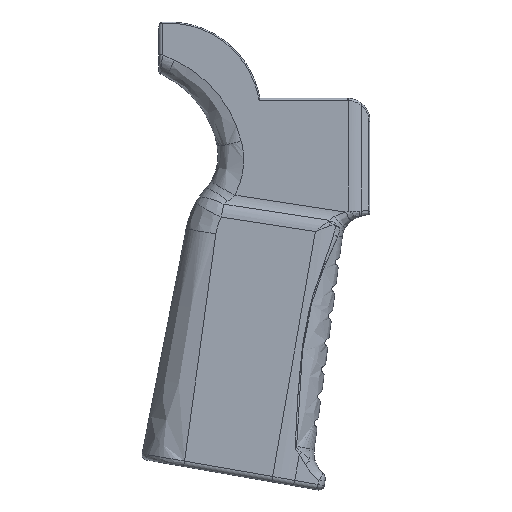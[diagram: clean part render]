
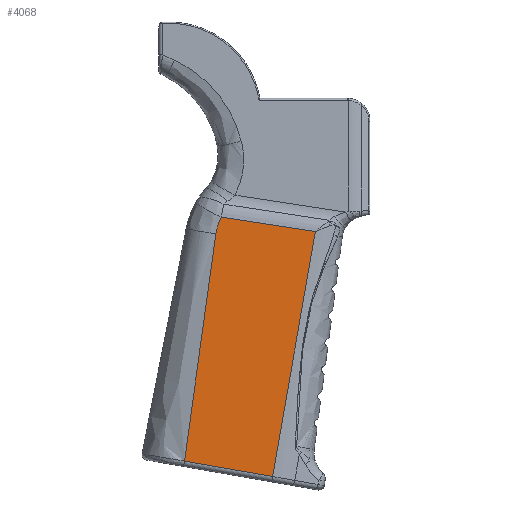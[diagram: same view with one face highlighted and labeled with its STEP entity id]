
A CAD part, left-side view. The second image highlights one B-rep face of the part: STEP entity #4068.
In plain terms, the highlighted planar face has unit normal (-1, 0, 0).
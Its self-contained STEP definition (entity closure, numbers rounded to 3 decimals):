
#224=PLANE('',#4393);
#483=FACE_OUTER_BOUND('',#751,.T.);
#751=EDGE_LOOP('',(#3697,#3698,#3699,#3700,#3701));
#1197=B_SPLINE_CURVE_WITH_KNOTS('',3,(#13325,#13326,#13327,#13328),
 .UNSPECIFIED.,.F.,.F.,(4,4),(6.533,7.017),
 .UNSPECIFIED.);
#1204=B_SPLINE_CURVE_WITH_KNOTS('',3,(#13594,#13595,#13596,#13597),
 .UNSPECIFIED.,.F.,.F.,(4,4),(0.175,6.533),
 .UNSPECIFIED.);
#1363=LINE('',#13222,#1530);
#1365=LINE('',#13591,#1532);
#1366=LINE('',#13593,#1533);
#1530=VECTOR('',#5151,10.);
#1532=VECTOR('',#5163,10.);
#1533=VECTOR('',#5166,10.);
#1831=VERTEX_POINT('',#11525);
#1880=VERTEX_POINT('',#12554);
#1899=VERTEX_POINT('',#13216);
#1903=VERTEX_POINT('',#13317);
#1906=VERTEX_POINT('',#13589);
#2499=EDGE_CURVE('',#1899,#1880,#1363,.T.);
#2506=EDGE_CURVE('',#1903,#1899,#1197,.T.);
#2515=EDGE_CURVE('',#1880,#1906,#1365,.T.);
#2516=EDGE_CURVE('',#1906,#1831,#1366,.T.);
#2517=EDGE_CURVE('',#1831,#1903,#1204,.T.);
#3697=ORIENTED_EDGE('',*,*,#2516,.F.);
#3698=ORIENTED_EDGE('',*,*,#2515,.F.);
#3699=ORIENTED_EDGE('',*,*,#2499,.F.);
#3700=ORIENTED_EDGE('',*,*,#2506,.F.);
#3701=ORIENTED_EDGE('',*,*,#2517,.F.);
#4068=ADVANCED_FACE('',(#483),#224,.F.);
#4393=AXIS2_PLACEMENT_3D('',#13592,#5164,#5165);
#5151=DIRECTION('',(0.,-0.989,-0.151));
#5163=DIRECTION('',(0.,0.172,-0.985));
#5164=DIRECTION('center_axis',(1.,0.,0.));
#5165=DIRECTION('ref_axis',(0.,-0.989,-0.151));
#5166=DIRECTION('',(0.,0.985,0.172));
#11525=CARTESIAN_POINT('',(11.668,-98.506,-71.96));
#12554=CARTESIAN_POINT('',(11.668,-134.704,-8.461));
#13216=CARTESIAN_POINT('',(11.668,-108.616,-4.478));
#13222=CARTESIAN_POINT('',(11.668,-118.173,-5.937));
#13317=CARTESIAN_POINT('',(11.668,-107.199,-9.084));
#13325=CARTESIAN_POINT('Ctrl Pts',(11.668,-107.199,-9.084));
#13326=CARTESIAN_POINT('Ctrl Pts',(11.668,-107.42,-7.486));
#13327=CARTESIAN_POINT('Ctrl Pts',(11.668,-107.902,-5.924));
#13328=CARTESIAN_POINT('Ctrl Pts',(11.668,-108.616,-4.478));
#13589=CARTESIAN_POINT('',(11.668,-122.882,-76.214));
#13591=CARTESIAN_POINT('',(11.668,-129.214,-39.923));
#13592=CARTESIAN_POINT('Origin',(11.668,-93.6,1.15));
#13593=CARTESIAN_POINT('',(11.668,-107.256,-73.487));
#13594=CARTESIAN_POINT('Ctrl Pts',(11.668,-98.506,-71.96));
#13595=CARTESIAN_POINT('Ctrl Pts',(11.668,-101.404,-50.999));
#13596=CARTESIAN_POINT('Ctrl Pts',(11.668,-104.301,-30.043));
#13597=CARTESIAN_POINT('Ctrl Pts',(11.668,-107.199,-9.084));
